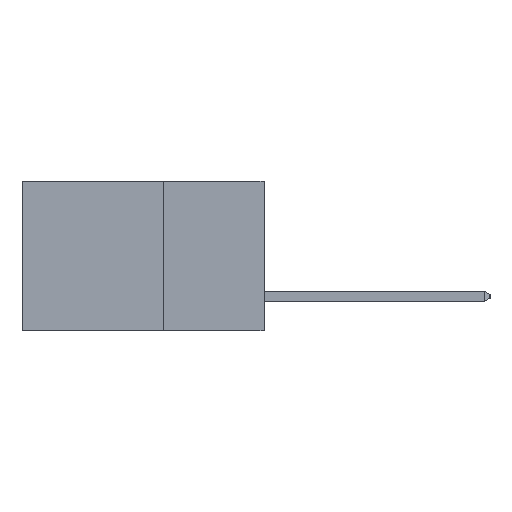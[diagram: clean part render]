
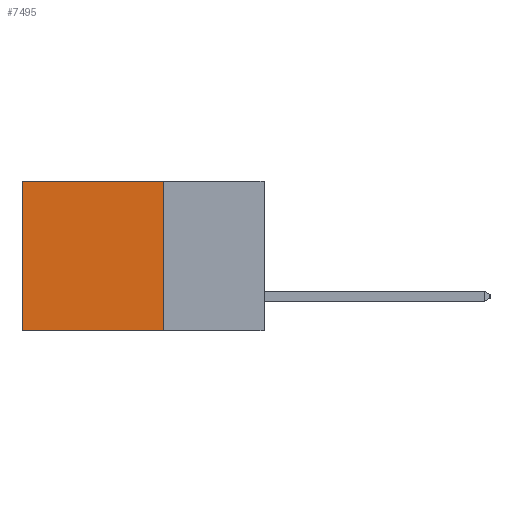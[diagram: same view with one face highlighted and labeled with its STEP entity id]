
A CAD part, left-side view. The second image highlights one B-rep face of the part: STEP entity #7495.
In plain terms, the highlighted planar face has unit normal (-1, 0, 0).
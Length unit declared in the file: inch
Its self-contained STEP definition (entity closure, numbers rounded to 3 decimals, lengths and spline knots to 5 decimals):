
#118 = DIRECTION ( 'NONE',  ( 0., 1., 0. ) ) ;
#304 = PLANE ( 'NONE',  #1949 ) ;
#531 = LINE ( 'NONE', #7403, #9600 ) ;
#848 = CARTESIAN_POINT ( 'NONE',  ( 0.2615, 0.25, 0. ) ) ;
#1138 = VECTOR ( 'NONE', #7451, 39.37008 ) ;
#1187 = ORIENTED_EDGE ( 'NONE', *, *, #2682, .T. ) ;
#1221 = DIRECTION ( 'NONE',  ( 0., 0., -1. ) ) ;
#1269 = CARTESIAN_POINT ( 'NONE',  ( 0.2615, 0.25, -0.37 ) ) ;
#1520 = EDGE_CURVE ( 'NONE', #7689, #8449, #10950, .T. ) ;
#1949 = AXIS2_PLACEMENT_3D ( 'NONE', #3942, #6514, #1221 ) ;
#2102 = DIRECTION ( 'NONE',  ( 0., 0., -1. ) ) ;
#2682 = EDGE_CURVE ( 'NONE', #4166, #8112, #7972, .T. ) ;
#3942 = CARTESIAN_POINT ( 'NONE',  ( 0.2615, 0.25, -0.37 ) ) ;
#4166 = VERTEX_POINT ( 'NONE', #4246 ) ;
#4194 = ORIENTED_EDGE ( 'NONE', *, *, #5938, .T. ) ;
#4246 = CARTESIAN_POINT ( 'NONE',  ( 0.2615, 0.6, 0. ) ) ;
#4466 = ORIENTED_EDGE ( 'NONE', *, *, #1520, .F. ) ;
#4696 = ORIENTED_EDGE ( 'NONE', *, *, #11034, .F. ) ;
#4912 = FACE_OUTER_BOUND ( 'NONE', #8417, .T. ) ;
#5058 = CARTESIAN_POINT ( 'NONE',  ( 0.2615, 0.25, 0. ) ) ;
#5938 = EDGE_CURVE ( 'NONE', #7689, #4166, #7892, .T. ) ;
#6514 = DIRECTION ( 'NONE',  ( 1., 0., 0. ) ) ;
#6768 = VECTOR ( 'NONE', #2102, 39.37008 ) ;
#7403 = CARTESIAN_POINT ( 'NONE',  ( 0.2615, 0.25, -0.37 ) ) ;
#7451 = DIRECTION ( 'NONE',  ( 0., 1., 0. ) ) ;
#7495 = ADVANCED_FACE ( 'NONE', ( #4912 ), #304, .F. ) ;
#7689 = VERTEX_POINT ( 'NONE', #5058 ) ;
#7892 = LINE ( 'NONE', #848, #1138 ) ;
#7972 = LINE ( 'NONE', #9101, #9957 ) ;
#8112 = VERTEX_POINT ( 'NONE', #8202 ) ;
#8202 = CARTESIAN_POINT ( 'NONE',  ( 0.2615, 0.6, -0.37 ) ) ;
#8417 = EDGE_LOOP ( 'NONE', ( #1187, #4696, #4466, #4194 ) ) ;
#8449 = VERTEX_POINT ( 'NONE', #11081 ) ;
#9101 = CARTESIAN_POINT ( 'NONE',  ( 0.2615, 0.6, -0.37 ) ) ;
#9600 = VECTOR ( 'NONE', #118, 39.37008 ) ;
#9957 = VECTOR ( 'NONE', #10481, 39.37008 ) ;
#10481 = DIRECTION ( 'NONE',  ( 0., 0., -1. ) ) ;
#10950 = LINE ( 'NONE', #1269, #6768 ) ;
#11034 = EDGE_CURVE ( 'NONE', #8449, #8112, #531, .T. ) ;
#11081 = CARTESIAN_POINT ( 'NONE',  ( 0.2615, 0.25, -0.37 ) ) ;
